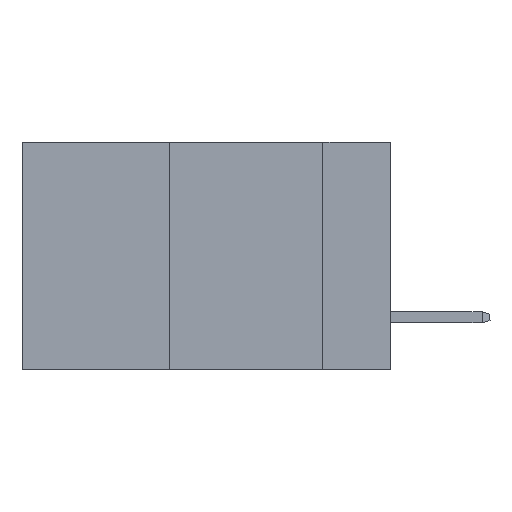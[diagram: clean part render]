
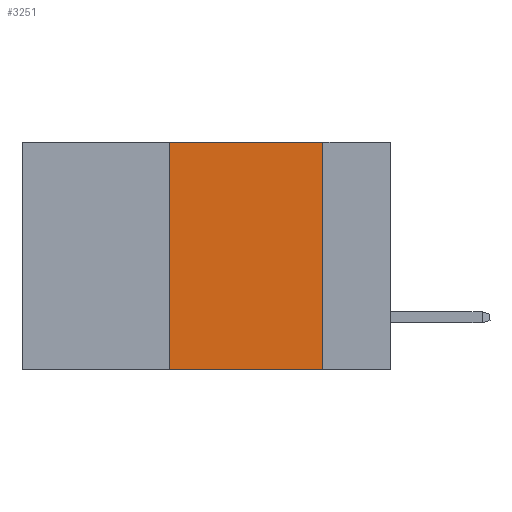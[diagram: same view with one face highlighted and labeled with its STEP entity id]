
A CAD part, left-side view. The second image highlights one B-rep face of the part: STEP entity #3251.
In plain terms, the highlighted planar face has unit normal (-1, 0, 0).
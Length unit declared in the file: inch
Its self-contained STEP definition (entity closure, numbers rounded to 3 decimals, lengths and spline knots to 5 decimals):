
#44 = ORIENTED_EDGE ( 'NONE', *, *, #21924, .F. ) ;
#561 = VECTOR ( 'NONE', #16744, 39.37008 ) ;
#607 = CARTESIAN_POINT ( 'NONE',  ( 0., 0.36, 0. ) ) ;
#1445 = LINE ( 'NONE', #13940, #28826 ) ;
#3251 = ADVANCED_FACE ( 'NONE', ( #28840 ), #14044, .F. ) ;
#3843 = VERTEX_POINT ( 'NONE', #607 ) ;
#4945 = CARTESIAN_POINT ( 'NONE',  ( 0., 0.11, 0. ) ) ;
#7052 = LINE ( 'NONE', #14065, #561 ) ;
#8705 = DIRECTION ( 'NONE',  ( 0., -1., 0. ) ) ;
#9122 = VECTOR ( 'NONE', #26818, 39.37008 ) ;
#9385 = EDGE_CURVE ( 'NONE', #11794, #26246, #29160, .T. ) ;
#11166 = CARTESIAN_POINT ( 'NONE',  ( 0., 0.6, -0.37 ) ) ;
#11242 = AXIS2_PLACEMENT_3D ( 'NONE', #21936, #29767, #14175 ) ;
#11472 = CARTESIAN_POINT ( 'NONE',  ( 0., 0.36, 0. ) ) ;
#11794 = VERTEX_POINT ( 'NONE', #24588 ) ;
#13940 = CARTESIAN_POINT ( 'NONE',  ( 0., 0.6, 0. ) ) ;
#13948 = ORIENTED_EDGE ( 'NONE', *, *, #9385, .T. ) ;
#14044 = PLANE ( 'NONE',  #11242 ) ;
#14065 = CARTESIAN_POINT ( 'NONE',  ( 0., 0.11, 0. ) ) ;
#14175 = DIRECTION ( 'NONE',  ( 0., 0., -1. ) ) ;
#14875 = EDGE_CURVE ( 'NONE', #11794, #3843, #21741, .T. ) ;
#16744 = DIRECTION ( 'NONE',  ( 0., 0., -1. ) ) ;
#19551 = EDGE_CURVE ( 'NONE', #22333, #26246, #7052, .T. ) ;
#20697 = ORIENTED_EDGE ( 'NONE', *, *, #14875, .F. ) ;
#21741 = LINE ( 'NONE', #11472, #27827 ) ;
#21924 = EDGE_CURVE ( 'NONE', #3843, #22333, #1445, .T. ) ;
#21936 = CARTESIAN_POINT ( 'NONE',  ( 0., 0.6, 0. ) ) ;
#22333 = VERTEX_POINT ( 'NONE', #4945 ) ;
#24588 = CARTESIAN_POINT ( 'NONE',  ( 0., 0.36, -0.37 ) ) ;
#26246 = VERTEX_POINT ( 'NONE', #32517 ) ;
#26818 = DIRECTION ( 'NONE',  ( 0., -1., 0. ) ) ;
#27415 = EDGE_LOOP ( 'NONE', ( #28844, #44, #20697, #13948 ) ) ;
#27827 = VECTOR ( 'NONE', #29741, 39.37008 ) ;
#28826 = VECTOR ( 'NONE', #8705, 39.37008 ) ;
#28840 = FACE_OUTER_BOUND ( 'NONE', #27415, .T. ) ;
#28844 = ORIENTED_EDGE ( 'NONE', *, *, #19551, .F. ) ;
#29160 = LINE ( 'NONE', #11166, #9122 ) ;
#29741 = DIRECTION ( 'NONE',  ( 0., 0., 1. ) ) ;
#29767 = DIRECTION ( 'NONE',  ( 1., 0., 0. ) ) ;
#32517 = CARTESIAN_POINT ( 'NONE',  ( 0., 0.11, -0.37 ) ) ;
